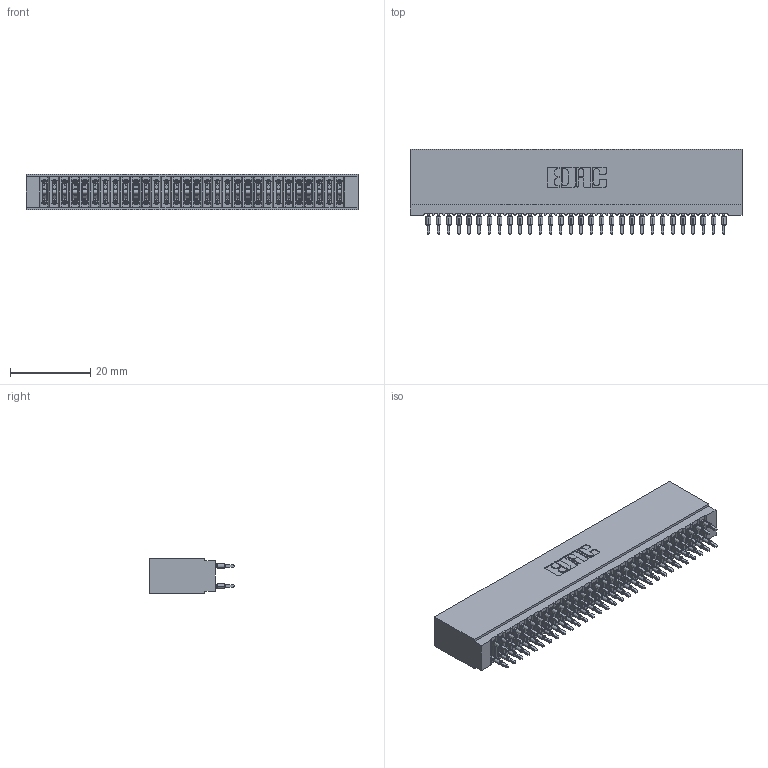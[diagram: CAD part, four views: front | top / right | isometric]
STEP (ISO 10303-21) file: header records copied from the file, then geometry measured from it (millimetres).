
FILE_DESCRIPTION (( 'STEP AP203' ), '1' );
FILE_NAME ('745-060-560-201.STEP', '2020-09-14T00:39:40', ( '' ), ( '' ), 'SwSTEP 2.0', 'SolidWorks 2020', '' );
FILE_SCHEMA (( 'CONFIG_CONTROL_DESIGN' ));
Length unit declared in the file: inch
Products named in the file (3): 745-060-560-201; 745-292-001_560; 745 Part_Insulator Option - 01
Assembly tree (61 placements, depth 2):
  745-060-560-201
    745 Part_Insulator Option - 01
    745-292-001_560  x60
Bounding box: 82.8 x 21.22 x 8.89 mm (x, y, z)
Volume: 7752 mm3; surface area: 16427.3 mm2
Topology: 61 solids, 61 shells, 6005 faces, 16428 edges, 10432 vertices
Faces by surface type: plane 3115, cylinder 1330, bspline 1200, torus 360
Entity records: 52473 total; most frequent: CARTESIAN_POINT 9609, ORIENTED_EDGE 9020, DIRECTION 7894, EDGE_CURVE 4510, LINE 4140, VECTOR 4140, VERTEX_POINT 2880, AXIS2_PLACEMENT_3D 1877
